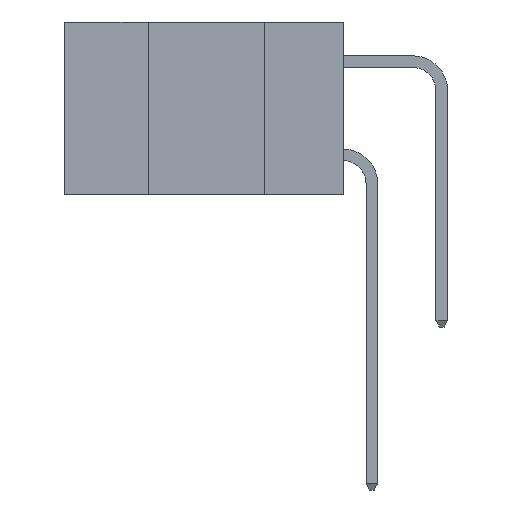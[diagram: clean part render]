
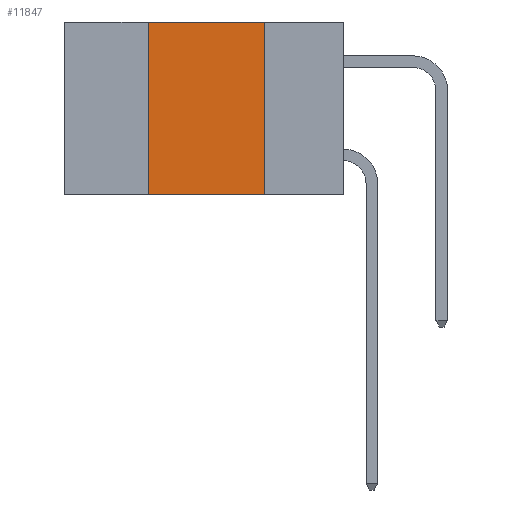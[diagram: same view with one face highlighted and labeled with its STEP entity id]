
A CAD part, left-side view. The second image highlights one B-rep face of the part: STEP entity #11847.
In plain terms, the highlighted planar face has unit normal (-1, 0, 0).
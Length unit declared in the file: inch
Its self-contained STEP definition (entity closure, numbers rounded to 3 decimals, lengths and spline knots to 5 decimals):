
#226 = CARTESIAN_POINT ( 'NONE',  ( 0., 0.17, -0.37 ) ) ;
#259 = EDGE_CURVE ( 'NONE', #19307, #13882, #3299, .T. ) ;
#1154 = CARTESIAN_POINT ( 'NONE',  ( 0., 0.6, 0. ) ) ;
#1662 = VERTEX_POINT ( 'NONE', #12092 ) ;
#2528 = CARTESIAN_POINT ( 'NONE',  ( 0., 0.6, -0.37 ) ) ;
#3299 = LINE ( 'NONE', #226, #17278 ) ;
#3571 = ORIENTED_EDGE ( 'NONE', *, *, #16781, .F. ) ;
#4518 = DIRECTION ( 'NONE',  ( 0., -1., 0. ) ) ;
#4573 = DIRECTION ( 'NONE',  ( 0., 0., -1. ) ) ;
#5060 = VECTOR ( 'NONE', #4518, 39.37008 ) ;
#5554 = PLANE ( 'NONE',  #10685 ) ;
#6876 = DIRECTION ( 'NONE',  ( 0., 0., 1. ) ) ;
#8975 = VECTOR ( 'NONE', #6876, 39.37008 ) ;
#9506 = CARTESIAN_POINT ( 'NONE',  ( 0., 0.42, 0. ) ) ;
#9889 = LINE ( 'NONE', #2528, #5060 ) ;
#10021 = EDGE_LOOP ( 'NONE', ( #16980, #3571, #18092, #18644 ) ) ;
#10685 = AXIS2_PLACEMENT_3D ( 'NONE', #21680, #11033, #23413 ) ;
#11033 = DIRECTION ( 'NONE',  ( 1., 0., 0. ) ) ;
#11847 = ADVANCED_FACE ( 'NONE', ( #20819 ), #5554, .F. ) ;
#12092 = CARTESIAN_POINT ( 'NONE',  ( 0., 0.42, -0.37 ) ) ;
#12591 = VERTEX_POINT ( 'NONE', #9506 ) ;
#12682 = VECTOR ( 'NONE', #17683, 39.37008 ) ;
#13882 = VERTEX_POINT ( 'NONE', #23200 ) ;
#14387 = LINE ( 'NONE', #17697, #8975 ) ;
#15018 = CARTESIAN_POINT ( 'NONE',  ( 0., 0.17, 0. ) ) ;
#15593 = EDGE_CURVE ( 'NONE', #1662, #13882, #9889, .T. ) ;
#16781 = EDGE_CURVE ( 'NONE', #12591, #19307, #17468, .T. ) ;
#16980 = ORIENTED_EDGE ( 'NONE', *, *, #259, .F. ) ;
#17278 = VECTOR ( 'NONE', #4573, 39.37008 ) ;
#17468 = LINE ( 'NONE', #1154, #12682 ) ;
#17683 = DIRECTION ( 'NONE',  ( 0., -1., 0. ) ) ;
#17697 = CARTESIAN_POINT ( 'NONE',  ( 0., 0.42, -0.37 ) ) ;
#18092 = ORIENTED_EDGE ( 'NONE', *, *, #20288, .F. ) ;
#18644 = ORIENTED_EDGE ( 'NONE', *, *, #15593, .T. ) ;
#19307 = VERTEX_POINT ( 'NONE', #15018 ) ;
#20288 = EDGE_CURVE ( 'NONE', #1662, #12591, #14387, .T. ) ;
#20819 = FACE_OUTER_BOUND ( 'NONE', #10021, .T. ) ;
#21680 = CARTESIAN_POINT ( 'NONE',  ( 0., 0.6, 0. ) ) ;
#23200 = CARTESIAN_POINT ( 'NONE',  ( 0., 0.17, -0.37 ) ) ;
#23413 = DIRECTION ( 'NONE',  ( 0., 0., -1. ) ) ;
